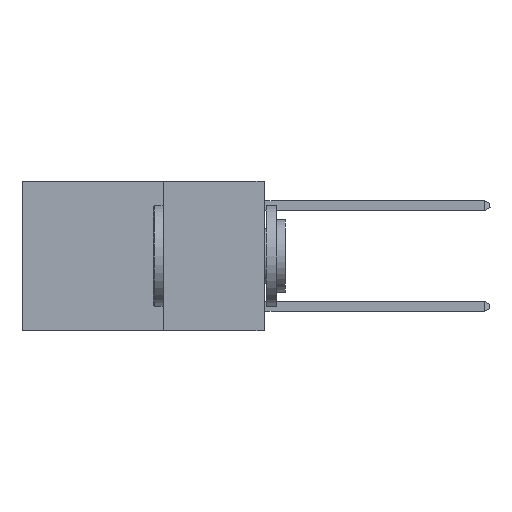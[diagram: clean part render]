
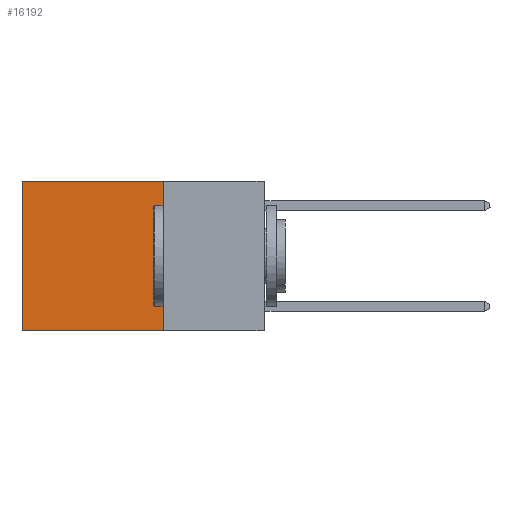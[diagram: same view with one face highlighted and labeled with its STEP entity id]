
A CAD part, left-side view. The second image highlights one B-rep face of the part: STEP entity #16192.
In plain terms, the highlighted planar face has unit normal (-1, 0, 0).
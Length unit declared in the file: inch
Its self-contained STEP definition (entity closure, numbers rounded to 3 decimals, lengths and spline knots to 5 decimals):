
#273 = EDGE_CURVE ( 'NONE', #6585, #17105, #11869, .T. ) ;
#670 = EDGE_LOOP ( 'NONE', ( #14809, #8256, #12404, #8514 ) ) ;
#764 = AXIS2_PLACEMENT_3D ( 'NONE', #7920, #12731, #3058 ) ;
#892 = CARTESIAN_POINT ( 'NONE',  ( 0.2625, 0.25, -0.37 ) ) ;
#2035 = VECTOR ( 'NONE', #6195, 39.37008 ) ;
#3058 = DIRECTION ( 'NONE',  ( 0., 0., -1. ) ) ;
#3164 = LINE ( 'NONE', #6907, #7962 ) ;
#3276 = FACE_OUTER_BOUND ( 'NONE', #670, .T. ) ;
#3400 = VERTEX_POINT ( 'NONE', #7863 ) ;
#4487 = VECTOR ( 'NONE', #10122, 39.37008 ) ;
#6038 = DIRECTION ( 'NONE',  ( 0., 1., 0. ) ) ;
#6195 = DIRECTION ( 'NONE',  ( 0., 0., -1. ) ) ;
#6585 = VERTEX_POINT ( 'NONE', #19273 ) ;
#6814 = EDGE_CURVE ( 'NONE', #3400, #15428, #3164, .T. ) ;
#6907 = CARTESIAN_POINT ( 'NONE',  ( 0.2625, 0.25, 0. ) ) ;
#7863 = CARTESIAN_POINT ( 'NONE',  ( 0.2625, 0.25, 0. ) ) ;
#7920 = CARTESIAN_POINT ( 'NONE',  ( 0.2625, 0.25, 0. ) ) ;
#7962 = VECTOR ( 'NONE', #13468, 39.37008 ) ;
#8256 = ORIENTED_EDGE ( 'NONE', *, *, #17132, .F. ) ;
#8514 = ORIENTED_EDGE ( 'NONE', *, *, #10921, .T. ) ;
#8925 = CARTESIAN_POINT ( 'NONE',  ( 0.2625, 0.6, -0.37 ) ) ;
#10122 = DIRECTION ( 'NONE',  ( 0., 1., 0. ) ) ;
#10640 = CARTESIAN_POINT ( 'NONE',  ( 0.2625, 0.25, -0.37 ) ) ;
#10806 = VECTOR ( 'NONE', #6038, 39.37008 ) ;
#10921 = EDGE_CURVE ( 'NONE', #3400, #6585, #15356, .T. ) ;
#11193 = CARTESIAN_POINT ( 'NONE',  ( 0.2625, 0.6, 0. ) ) ;
#11869 = LINE ( 'NONE', #11193, #2035 ) ;
#12404 = ORIENTED_EDGE ( 'NONE', *, *, #6814, .F. ) ;
#12525 = PLANE ( 'NONE',  #764 ) ;
#12731 = DIRECTION ( 'NONE',  ( 1., 0., 0. ) ) ;
#13468 = DIRECTION ( 'NONE',  ( 0., 0., -1. ) ) ;
#13574 = CARTESIAN_POINT ( 'NONE',  ( 0.2625, 0.25, 0. ) ) ;
#14809 = ORIENTED_EDGE ( 'NONE', *, *, #273, .T. ) ;
#15356 = LINE ( 'NONE', #13574, #4487 ) ;
#15428 = VERTEX_POINT ( 'NONE', #10640 ) ;
#16192 = ADVANCED_FACE ( 'NONE', ( #3276 ), #12525, .F. ) ;
#17105 = VERTEX_POINT ( 'NONE', #8925 ) ;
#17132 = EDGE_CURVE ( 'NONE', #15428, #17105, #18302, .T. ) ;
#18302 = LINE ( 'NONE', #892, #10806 ) ;
#19273 = CARTESIAN_POINT ( 'NONE',  ( 0.2625, 0.6, 0. ) ) ;
